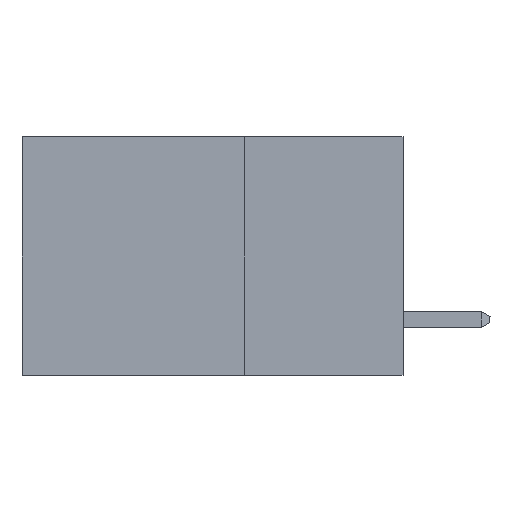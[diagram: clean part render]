
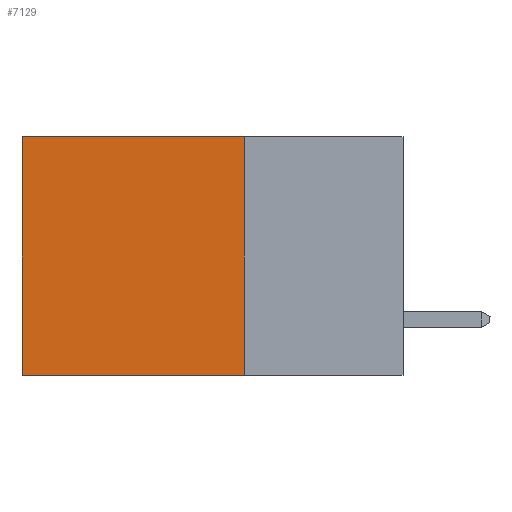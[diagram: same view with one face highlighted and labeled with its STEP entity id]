
A CAD part, left-side view. The second image highlights one B-rep face of the part: STEP entity #7129.
In plain terms, the highlighted planar face has unit normal (-1, 0, 0).
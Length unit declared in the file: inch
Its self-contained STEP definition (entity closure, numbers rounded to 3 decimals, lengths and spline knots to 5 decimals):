
#202 = AXIS2_PLACEMENT_3D ( 'NONE', #14023, #9472, #8052 ) ;
#235 = VERTEX_POINT ( 'NONE', #12601 ) ;
#774 = ORIENTED_EDGE ( 'NONE', *, *, #1359, .T. ) ;
#783 = VECTOR ( 'NONE', #7303, 39.37008 ) ;
#1359 = EDGE_CURVE ( 'NONE', #5716, #3655, #6162, .T. ) ;
#1593 = VECTOR ( 'NONE', #8365, 39.37008 ) ;
#1742 = CARTESIAN_POINT ( 'NONE',  ( 0.2875, 0.25, 0. ) ) ;
#1871 = CARTESIAN_POINT ( 'NONE',  ( 0.2875, 0.6, -0.375 ) ) ;
#3179 = EDGE_CURVE ( 'NONE', #3655, #235, #17679, .T. ) ;
#3655 = VERTEX_POINT ( 'NONE', #11935 ) ;
#5399 = CARTESIAN_POINT ( 'NONE',  ( 0.2875, 0.25, -0.375 ) ) ;
#5694 = VECTOR ( 'NONE', #6273, 39.37008 ) ;
#5716 = VERTEX_POINT ( 'NONE', #1742 ) ;
#5882 = VECTOR ( 'NONE', #9267, 39.37008 ) ;
#6162 = LINE ( 'NONE', #18102, #5694 ) ;
#6273 = DIRECTION ( 'NONE',  ( 0., 1., 0. ) ) ;
#6513 = PLANE ( 'NONE',  #202 ) ;
#7129 = ADVANCED_FACE ( 'NONE', ( #12783 ), #6513, .F. ) ;
#7303 = DIRECTION ( 'NONE',  ( 0., 1., 0. ) ) ;
#7426 = CARTESIAN_POINT ( 'NONE',  ( 0.2875, 0.25, -0.375 ) ) ;
#8052 = DIRECTION ( 'NONE',  ( 0., 0., -1. ) ) ;
#8365 = DIRECTION ( 'NONE',  ( 0., 0., -1. ) ) ;
#8684 = EDGE_CURVE ( 'NONE', #18665, #235, #15325, .T. ) ;
#9267 = DIRECTION ( 'NONE',  ( 0., 0., -1. ) ) ;
#9472 = DIRECTION ( 'NONE',  ( 1., 0., 0. ) ) ;
#11103 = ORIENTED_EDGE ( 'NONE', *, *, #3179, .T. ) ;
#11935 = CARTESIAN_POINT ( 'NONE',  ( 0.2875, 0.6, 0. ) ) ;
#12507 = ORIENTED_EDGE ( 'NONE', *, *, #8684, .F. ) ;
#12601 = CARTESIAN_POINT ( 'NONE',  ( 0.2875, 0.6, -0.375 ) ) ;
#12783 = FACE_OUTER_BOUND ( 'NONE', #15084, .T. ) ;
#13293 = EDGE_CURVE ( 'NONE', #5716, #18665, #16148, .T. ) ;
#14023 = CARTESIAN_POINT ( 'NONE',  ( 0.2875, 0.25, -0.375 ) ) ;
#14065 = CARTESIAN_POINT ( 'NONE',  ( 0.2875, 0.25, -0.375 ) ) ;
#15084 = EDGE_LOOP ( 'NONE', ( #11103, #12507, #17709, #774 ) ) ;
#15325 = LINE ( 'NONE', #7426, #783 ) ;
#16148 = LINE ( 'NONE', #5399, #1593 ) ;
#17679 = LINE ( 'NONE', #1871, #5882 ) ;
#17709 = ORIENTED_EDGE ( 'NONE', *, *, #13293, .F. ) ;
#18102 = CARTESIAN_POINT ( 'NONE',  ( 0.2875, 0.25, 0. ) ) ;
#18665 = VERTEX_POINT ( 'NONE', #14065 ) ;
